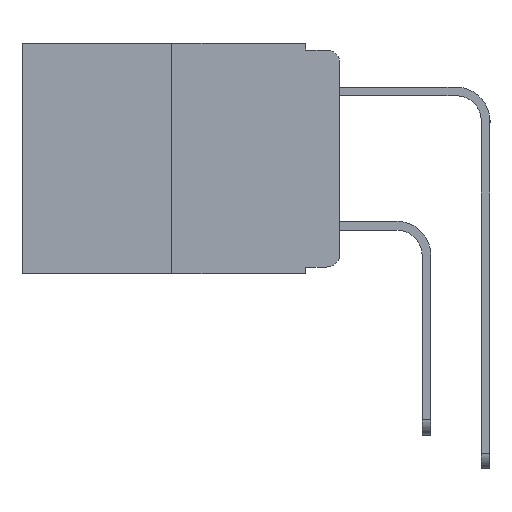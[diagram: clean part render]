
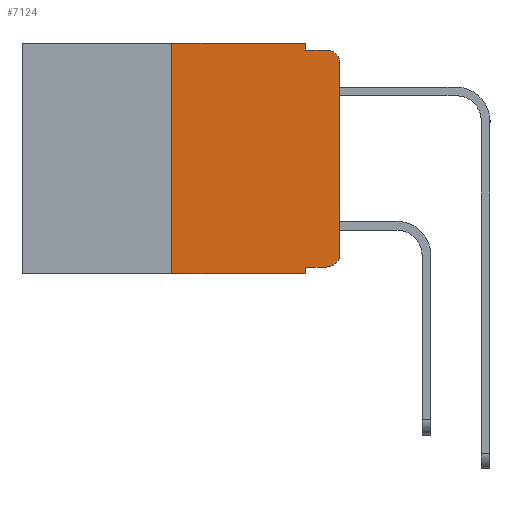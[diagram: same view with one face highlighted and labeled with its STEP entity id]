
A CAD part, left-side view. The second image highlights one B-rep face of the part: STEP entity #7124.
In plain terms, the highlighted planar face has unit normal (-1, 0, 0).
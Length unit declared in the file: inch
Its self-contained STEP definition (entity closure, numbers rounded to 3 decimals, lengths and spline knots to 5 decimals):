
#253 = LINE ( 'NONE', #5229, #13944 ) ;
#560 = ORIENTED_EDGE ( 'NONE', *, *, #5237, .F. ) ;
#686 = AXIS2_PLACEMENT_3D ( 'NONE', #6222, #18106, #7948 ) ;
#1146 = ORIENTED_EDGE ( 'NONE', *, *, #2971, .F. ) ;
#1647 = CARTESIAN_POINT ( 'NONE',  ( 0., 0.02, -0.01 ) ) ;
#1729 = CARTESIAN_POINT ( 'NONE',  ( 0., 0., 0. ) ) ;
#1744 = AXIS2_PLACEMENT_3D ( 'NONE', #19443, #9393, #21090 ) ;
#1800 = EDGE_CURVE ( 'NONE', #6699, #20319, #253, .T. ) ;
#2301 = AXIS2_PLACEMENT_3D ( 'NONE', #3540, #5279, #17154 ) ;
#2387 = CARTESIAN_POINT ( 'NONE',  ( 0., 0.051, -0.333 ) ) ;
#2548 = DIRECTION ( 'NONE',  ( 0., 0., 1. ) ) ;
#2971 = EDGE_CURVE ( 'NONE', #16202, #7507, #21419, .T. ) ;
#3074 = DIRECTION ( 'NONE',  ( 0., -1., 0. ) ) ;
#3231 = DIRECTION ( 'NONE',  ( 0., -1., 0. ) ) ;
#3540 = CARTESIAN_POINT ( 'NONE',  ( 0., 0.473, 0. ) ) ;
#3582 = EDGE_LOOP ( 'NONE', ( #8624, #13160, #18173, #560, #18681, #1146, #5694, #6223, #20191, #7290 ) ) ;
#3889 = LINE ( 'NONE', #11769, #12410 ) ;
#3942 = CARTESIAN_POINT ( 'NONE',  ( 0., 0., -0.03 ) ) ;
#4010 = VECTOR ( 'NONE', #2548, 39.37008 ) ;
#4029 = CARTESIAN_POINT ( 'NONE',  ( 0., 0.051, -0.333 ) ) ;
#4378 = EDGE_CURVE ( 'NONE', #16202, #20319, #11426, .T. ) ;
#4653 = CIRCLE ( 'NONE', #686, 0.02 ) ;
#5229 = CARTESIAN_POINT ( 'NONE',  ( 0., 0.051, 0. ) ) ;
#5230 = VECTOR ( 'NONE', #15345, 39.37008 ) ;
#5237 = EDGE_CURVE ( 'NONE', #8317, #13177, #12428, .T. ) ;
#5254 = VECTOR ( 'NONE', #12362, 39.37008 ) ;
#5279 = DIRECTION ( 'NONE',  ( 1., 0., 0. ) ) ;
#5694 = ORIENTED_EDGE ( 'NONE', *, *, #4378, .T. ) ;
#5724 = DIRECTION ( 'NONE',  ( 0., 0., -1. ) ) ;
#5933 = CARTESIAN_POINT ( 'NONE',  ( 0., 0.02, -0.333 ) ) ;
#6222 = CARTESIAN_POINT ( 'NONE',  ( 0., 0.02, -0.03 ) ) ;
#6223 = ORIENTED_EDGE ( 'NONE', *, *, #1800, .F. ) ;
#6368 = EDGE_CURVE ( 'NONE', #13177, #6395, #3889, .T. ) ;
#6395 = VERTEX_POINT ( 'NONE', #1647 ) ;
#6699 = VERTEX_POINT ( 'NONE', #2387 ) ;
#7124 = ADVANCED_FACE ( 'NONE', ( #7584 ), #13773, .F. ) ;
#7290 = ORIENTED_EDGE ( 'NONE', *, *, #18174, .T. ) ;
#7504 = EDGE_CURVE ( 'NONE', #8572, #6395, #4653, .T. ) ;
#7507 = VERTEX_POINT ( 'NONE', #16410 ) ;
#7584 = FACE_OUTER_BOUND ( 'NONE', #3582, .T. ) ;
#7926 = VECTOR ( 'NONE', #5724, 39.37008 ) ;
#7948 = DIRECTION ( 'NONE',  ( 0., 0., -1. ) ) ;
#8317 = VERTEX_POINT ( 'NONE', #8438 ) ;
#8438 = CARTESIAN_POINT ( 'NONE',  ( 0., 0.051, 0. ) ) ;
#8572 = VERTEX_POINT ( 'NONE', #3942 ) ;
#8624 = ORIENTED_EDGE ( 'NONE', *, *, #10946, .T. ) ;
#9138 = CARTESIAN_POINT ( 'NONE',  ( 0., 0.051, -0.01 ) ) ;
#9393 = DIRECTION ( 'NONE',  ( -1., 0., 0. ) ) ;
#9914 = VERTEX_POINT ( 'NONE', #17444 ) ;
#10308 = LINE ( 'NONE', #1729, #5230 ) ;
#10886 = VECTOR ( 'NONE', #3074, 39.37008 ) ;
#10946 = EDGE_CURVE ( 'NONE', #9914, #8572, #10308, .T. ) ;
#11027 = CARTESIAN_POINT ( 'NONE',  ( 0., 0.25, 0. ) ) ;
#11426 = LINE ( 'NONE', #18287, #10886 ) ;
#11769 = CARTESIAN_POINT ( 'NONE',  ( 0., 0.051, -0.01 ) ) ;
#11921 = VERTEX_POINT ( 'NONE', #5933 ) ;
#12362 = DIRECTION ( 'NONE',  ( 0., -1., 0. ) ) ;
#12410 = VECTOR ( 'NONE', #3231, 39.37008 ) ;
#12428 = LINE ( 'NONE', #14221, #7926 ) ;
#13160 = ORIENTED_EDGE ( 'NONE', *, *, #7504, .T. ) ;
#13177 = VERTEX_POINT ( 'NONE', #9138 ) ;
#13773 = PLANE ( 'NONE',  #2301 ) ;
#13944 = VECTOR ( 'NONE', #17112, 39.37008 ) ;
#14221 = CARTESIAN_POINT ( 'NONE',  ( 0., 0.051, 0. ) ) ;
#14311 = LINE ( 'NONE', #15727, #5254 ) ;
#15345 = DIRECTION ( 'NONE',  ( 0., 0., 1. ) ) ;
#15577 = CARTESIAN_POINT ( 'NONE',  ( 0., 0.051, -0.343 ) ) ;
#15727 = CARTESIAN_POINT ( 'NONE',  ( 0., 0.473, 0. ) ) ;
#16202 = VERTEX_POINT ( 'NONE', #17486 ) ;
#16410 = CARTESIAN_POINT ( 'NONE',  ( 0., 0.25, 0. ) ) ;
#16466 = CIRCLE ( 'NONE', #1744, 0.02 ) ;
#16679 = LINE ( 'NONE', #4029, #20519 ) ;
#17112 = DIRECTION ( 'NONE',  ( 0., 0., -1. ) ) ;
#17154 = DIRECTION ( 'NONE',  ( 0., 0., -1. ) ) ;
#17444 = CARTESIAN_POINT ( 'NONE',  ( 0., 0., -0.313 ) ) ;
#17486 = CARTESIAN_POINT ( 'NONE',  ( 0., 0.25, -0.343 ) ) ;
#18106 = DIRECTION ( 'NONE',  ( -1., 0., 0. ) ) ;
#18173 = ORIENTED_EDGE ( 'NONE', *, *, #6368, .F. ) ;
#18174 = EDGE_CURVE ( 'NONE', #11921, #9914, #16466, .T. ) ;
#18287 = CARTESIAN_POINT ( 'NONE',  ( 0., 0.473, -0.343 ) ) ;
#18681 = ORIENTED_EDGE ( 'NONE', *, *, #19157, .F. ) ;
#19157 = EDGE_CURVE ( 'NONE', #7507, #8317, #14311, .T. ) ;
#19240 = EDGE_CURVE ( 'NONE', #6699, #11921, #16679, .T. ) ;
#19262 = DIRECTION ( 'NONE',  ( 0., -1., 0. ) ) ;
#19443 = CARTESIAN_POINT ( 'NONE',  ( 0., 0.02, -0.313 ) ) ;
#20191 = ORIENTED_EDGE ( 'NONE', *, *, #19240, .T. ) ;
#20319 = VERTEX_POINT ( 'NONE', #15577 ) ;
#20519 = VECTOR ( 'NONE', #19262, 39.37008 ) ;
#21090 = DIRECTION ( 'NONE',  ( 0., 0., -1. ) ) ;
#21419 = LINE ( 'NONE', #11027, #4010 ) ;
